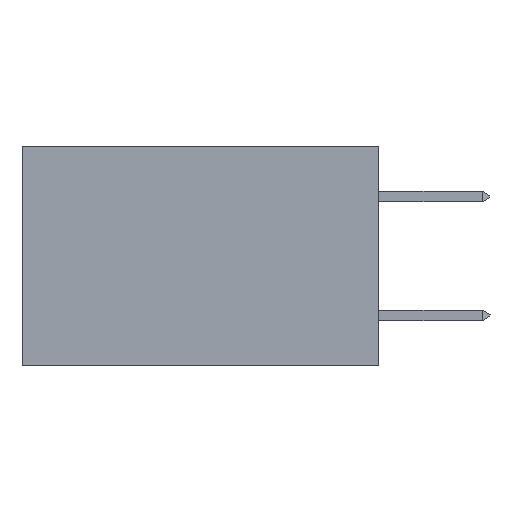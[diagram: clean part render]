
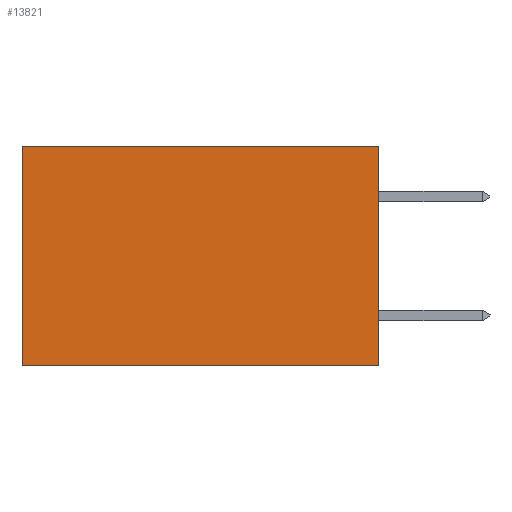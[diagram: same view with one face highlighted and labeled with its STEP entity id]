
A CAD part, left-side view. The second image highlights one B-rep face of the part: STEP entity #13821.
In plain terms, the highlighted planar face has unit normal (-1, 0, 0).
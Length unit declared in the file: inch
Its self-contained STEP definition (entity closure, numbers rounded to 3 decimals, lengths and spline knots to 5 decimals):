
#50 = DIRECTION ( 'NONE',  ( 0., 1., 0. ) ) ;
#233 = VERTEX_POINT ( 'NONE', #13382 ) ;
#495 = VECTOR ( 'NONE', #4214, 39.37008 ) ;
#1099 = PLANE ( 'NONE',  #8956 ) ;
#2462 = DIRECTION ( 'NONE',  ( 0., 0., -1. ) ) ;
#2485 = DIRECTION ( 'NONE',  ( 0., 1., 0. ) ) ;
#3174 = CARTESIAN_POINT ( 'NONE',  ( 0.298, 0., -0.37 ) ) ;
#4214 = DIRECTION ( 'NONE',  ( 0., 0., -1. ) ) ;
#5239 = VECTOR ( 'NONE', #2462, 39.37008 ) ;
#5517 = EDGE_CURVE ( 'NONE', #14825, #10847, #12030, .T. ) ;
#5536 = ORIENTED_EDGE ( 'NONE', *, *, #11186, .T. ) ;
#5876 = EDGE_LOOP ( 'NONE', ( #5536, #13440, #14142, #15380 ) ) ;
#5891 = DIRECTION ( 'NONE',  ( 1., 0., 0. ) ) ;
#6103 = VECTOR ( 'NONE', #2485, 39.37008 ) ;
#6302 = CARTESIAN_POINT ( 'NONE',  ( 0.298, 0., 0. ) ) ;
#7183 = CARTESIAN_POINT ( 'NONE',  ( 0.298, 0.6, 0. ) ) ;
#8196 = CARTESIAN_POINT ( 'NONE',  ( 0.298, 0., 0. ) ) ;
#8285 = CARTESIAN_POINT ( 'NONE',  ( 0.298, 0., -0.37 ) ) ;
#8402 = LINE ( 'NONE', #7183, #5239 ) ;
#8949 = LINE ( 'NONE', #6302, #11414 ) ;
#8956 = AXIS2_PLACEMENT_3D ( 'NONE', #10827, #5891, #9542 ) ;
#9542 = DIRECTION ( 'NONE',  ( 0., 0., -1. ) ) ;
#10827 = CARTESIAN_POINT ( 'NONE',  ( 0.298, 0., 0. ) ) ;
#10847 = VERTEX_POINT ( 'NONE', #3174 ) ;
#10899 = CARTESIAN_POINT ( 'NONE',  ( 0.298, 0.6, -0.37 ) ) ;
#11186 = EDGE_CURVE ( 'NONE', #233, #12678, #8402, .T. ) ;
#11414 = VECTOR ( 'NONE', #50, 39.37008 ) ;
#12030 = LINE ( 'NONE', #8196, #495 ) ;
#12124 = FACE_OUTER_BOUND ( 'NONE', #5876, .T. ) ;
#12365 = EDGE_CURVE ( 'NONE', #14825, #233, #8949, .T. ) ;
#12505 = LINE ( 'NONE', #8285, #6103 ) ;
#12678 = VERTEX_POINT ( 'NONE', #10899 ) ;
#12962 = CARTESIAN_POINT ( 'NONE',  ( 0.298, 0., 0. ) ) ;
#13382 = CARTESIAN_POINT ( 'NONE',  ( 0.298, 0.6, 0. ) ) ;
#13440 = ORIENTED_EDGE ( 'NONE', *, *, #13865, .F. ) ;
#13821 = ADVANCED_FACE ( 'NONE', ( #12124 ), #1099, .F. ) ;
#13865 = EDGE_CURVE ( 'NONE', #10847, #12678, #12505, .T. ) ;
#14142 = ORIENTED_EDGE ( 'NONE', *, *, #5517, .F. ) ;
#14825 = VERTEX_POINT ( 'NONE', #12962 ) ;
#15380 = ORIENTED_EDGE ( 'NONE', *, *, #12365, .T. ) ;
